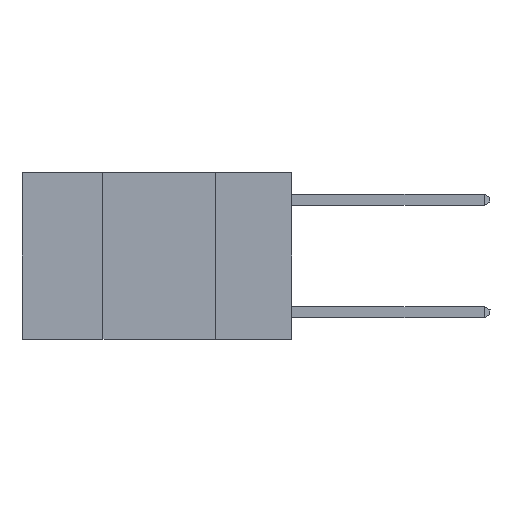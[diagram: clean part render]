
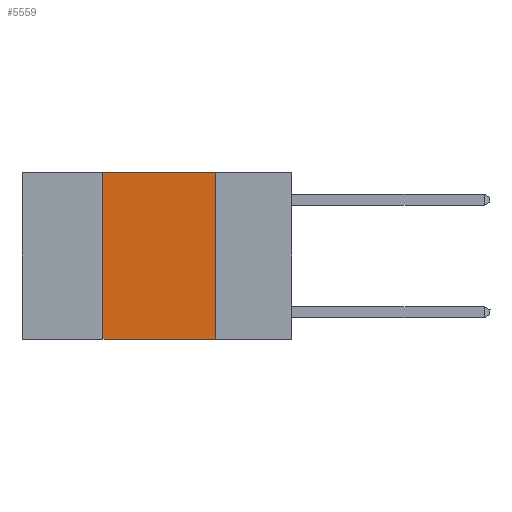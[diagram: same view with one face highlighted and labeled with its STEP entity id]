
A CAD part, left-side view. The second image highlights one B-rep face of the part: STEP entity #5559.
In plain terms, the highlighted planar face has unit normal (-1, 0, 0).
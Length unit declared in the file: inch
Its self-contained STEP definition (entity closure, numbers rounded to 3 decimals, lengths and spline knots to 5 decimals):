
#547 = DIRECTION ( 'NONE',  ( 0., 0., -1. ) ) ;
#659 = DIRECTION ( 'NONE',  ( 0., -1., 0. ) ) ;
#719 = EDGE_CURVE ( 'NONE', #7926, #11040, #8050, .T. ) ;
#964 = CARTESIAN_POINT ( 'NONE',  ( 0., 0.42, 0. ) ) ;
#1089 = FACE_OUTER_BOUND ( 'NONE', #4647, .T. ) ;
#1294 = ORIENTED_EDGE ( 'NONE', *, *, #9975, .F. ) ;
#1565 = CARTESIAN_POINT ( 'NONE',  ( 0., 0.6, -0.37 ) ) ;
#1744 = DIRECTION ( 'NONE',  ( 1., 0., 0. ) ) ;
#2662 = ORIENTED_EDGE ( 'NONE', *, *, #719, .T. ) ;
#3057 = AXIS2_PLACEMENT_3D ( 'NONE', #10624, #1744, #8049 ) ;
#3664 = CARTESIAN_POINT ( 'NONE',  ( 0., 0.42, 0. ) ) ;
#4086 = VECTOR ( 'NONE', #4973, 39.37008 ) ;
#4365 = LINE ( 'NONE', #11216, #4086 ) ;
#4401 = VECTOR ( 'NONE', #547, 39.37008 ) ;
#4647 = EDGE_LOOP ( 'NONE', ( #10282, #10036, #1294, #2662 ) ) ;
#4973 = DIRECTION ( 'NONE',  ( 0., -1., 0. ) ) ;
#5325 = DIRECTION ( 'NONE',  ( 0., 0., 1. ) ) ;
#5559 = ADVANCED_FACE ( 'NONE', ( #1089 ), #7093, .F. ) ;
#5646 = VECTOR ( 'NONE', #659, 39.37008 ) ;
#5835 = VERTEX_POINT ( 'NONE', #7612 ) ;
#5880 = CARTESIAN_POINT ( 'NONE',  ( 0., 0.17, 0. ) ) ;
#6445 = CARTESIAN_POINT ( 'NONE',  ( 0., 0.42, -0.37 ) ) ;
#7093 = PLANE ( 'NONE',  #3057 ) ;
#7612 = CARTESIAN_POINT ( 'NONE',  ( 0., 0.17, 0. ) ) ;
#7926 = VERTEX_POINT ( 'NONE', #6445 ) ;
#8049 = DIRECTION ( 'NONE',  ( 0., 0., -1. ) ) ;
#8050 = LINE ( 'NONE', #1565, #5646 ) ;
#8261 = VECTOR ( 'NONE', #5325, 39.37008 ) ;
#9261 = LINE ( 'NONE', #5880, #4401 ) ;
#9628 = EDGE_CURVE ( 'NONE', #5835, #11040, #9261, .T. ) ;
#9975 = EDGE_CURVE ( 'NONE', #7926, #10828, #10304, .T. ) ;
#10036 = ORIENTED_EDGE ( 'NONE', *, *, #11168, .F. ) ;
#10178 = CARTESIAN_POINT ( 'NONE',  ( 0., 0.17, -0.37 ) ) ;
#10282 = ORIENTED_EDGE ( 'NONE', *, *, #9628, .F. ) ;
#10304 = LINE ( 'NONE', #964, #8261 ) ;
#10624 = CARTESIAN_POINT ( 'NONE',  ( 0., 0.6, 0. ) ) ;
#10828 = VERTEX_POINT ( 'NONE', #3664 ) ;
#11040 = VERTEX_POINT ( 'NONE', #10178 ) ;
#11168 = EDGE_CURVE ( 'NONE', #10828, #5835, #4365, .T. ) ;
#11216 = CARTESIAN_POINT ( 'NONE',  ( 0., 0.6, 0. ) ) ;
